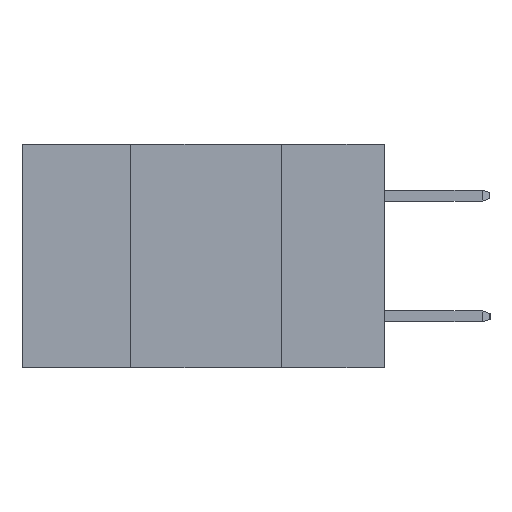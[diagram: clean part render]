
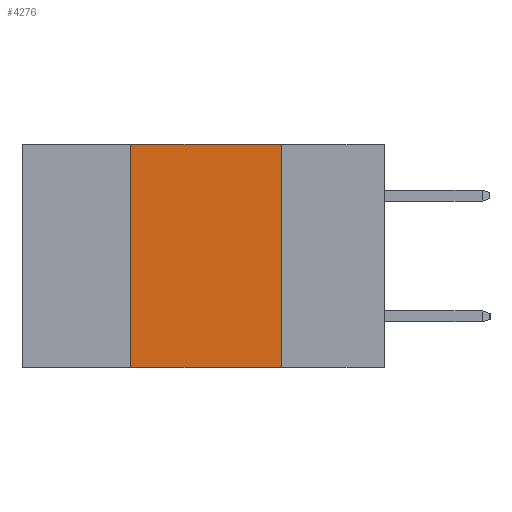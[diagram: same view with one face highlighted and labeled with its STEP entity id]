
A CAD part, left-side view. The second image highlights one B-rep face of the part: STEP entity #4276.
In plain terms, the highlighted planar face has unit normal (-1, 0, 0).
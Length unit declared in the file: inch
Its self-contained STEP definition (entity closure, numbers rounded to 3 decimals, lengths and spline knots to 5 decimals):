
#381 = VERTEX_POINT ( 'NONE', #8181 ) ;
#1112 = CARTESIAN_POINT ( 'NONE',  ( 0., 0.42, -0.37 ) ) ;
#1121 = CARTESIAN_POINT ( 'NONE',  ( 0., 0.17, -0.37 ) ) ;
#1545 = ORIENTED_EDGE ( 'NONE', *, *, #9450, .F. ) ;
#2863 = EDGE_CURVE ( 'NONE', #11625, #381, #8786, .T. ) ;
#2972 = ORIENTED_EDGE ( 'NONE', *, *, #2863, .F. ) ;
#3084 = DIRECTION ( 'NONE',  ( 0., -1., 0. ) ) ;
#3238 = LINE ( 'NONE', #1121, #10021 ) ;
#4096 = VERTEX_POINT ( 'NONE', #5447 ) ;
#4276 = ADVANCED_FACE ( 'NONE', ( #11046 ), #7323, .F. ) ;
#4389 = CARTESIAN_POINT ( 'NONE',  ( 0., 0.6, 0. ) ) ;
#4433 = VECTOR ( 'NONE', #3084, 39.37008 ) ;
#4578 = DIRECTION ( 'NONE',  ( 1., 0., 0. ) ) ;
#4701 = EDGE_LOOP ( 'NONE', ( #8752, #2972, #1545, #11372 ) ) ;
#5447 = CARTESIAN_POINT ( 'NONE',  ( 0., 0.42, -0.37 ) ) ;
#5925 = VECTOR ( 'NONE', #9126, 39.37008 ) ;
#7323 = PLANE ( 'NONE',  #7325 ) ;
#7325 = AXIS2_PLACEMENT_3D ( 'NONE', #4389, #4578, #7983 ) ;
#7606 = CARTESIAN_POINT ( 'NONE',  ( 0., 0.42, 0. ) ) ;
#7983 = DIRECTION ( 'NONE',  ( 0., 0., -1. ) ) ;
#8181 = CARTESIAN_POINT ( 'NONE',  ( 0., 0.17, 0. ) ) ;
#8465 = CARTESIAN_POINT ( 'NONE',  ( 0., 0.6, -0.37 ) ) ;
#8752 = ORIENTED_EDGE ( 'NONE', *, *, #11785, .F. ) ;
#8786 = LINE ( 'NONE', #9088, #5925 ) ;
#9088 = CARTESIAN_POINT ( 'NONE',  ( 0., 0.6, 0. ) ) ;
#9126 = DIRECTION ( 'NONE',  ( 0., -1., 0. ) ) ;
#9450 = EDGE_CURVE ( 'NONE', #4096, #11625, #11692, .T. ) ;
#9475 = DIRECTION ( 'NONE',  ( 0., 0., 1. ) ) ;
#9590 = VECTOR ( 'NONE', #9475, 39.37008 ) ;
#10021 = VECTOR ( 'NONE', #10304, 39.37008 ) ;
#10304 = DIRECTION ( 'NONE',  ( 0., 0., -1. ) ) ;
#10560 = VERTEX_POINT ( 'NONE', #11582 ) ;
#11046 = FACE_OUTER_BOUND ( 'NONE', #4701, .T. ) ;
#11262 = LINE ( 'NONE', #8465, #4433 ) ;
#11372 = ORIENTED_EDGE ( 'NONE', *, *, #11584, .T. ) ;
#11582 = CARTESIAN_POINT ( 'NONE',  ( 0., 0.17, -0.37 ) ) ;
#11584 = EDGE_CURVE ( 'NONE', #4096, #10560, #11262, .T. ) ;
#11625 = VERTEX_POINT ( 'NONE', #7606 ) ;
#11692 = LINE ( 'NONE', #1112, #9590 ) ;
#11785 = EDGE_CURVE ( 'NONE', #381, #10560, #3238, .T. ) ;
